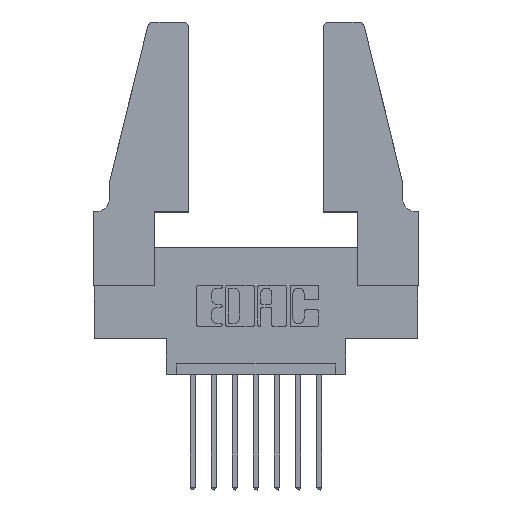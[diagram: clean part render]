
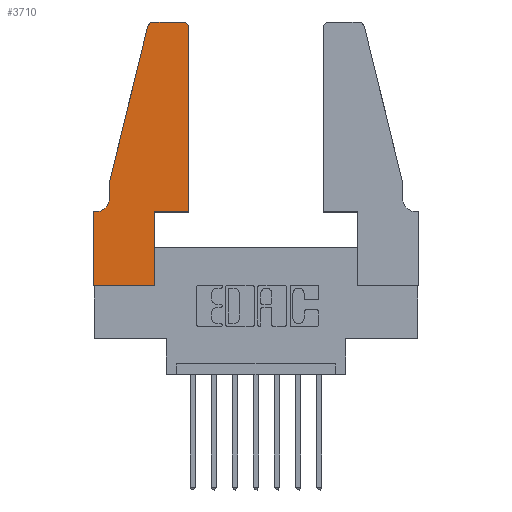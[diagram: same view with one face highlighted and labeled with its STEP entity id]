
A CAD part, top view. The second image highlights one B-rep face of the part: STEP entity #3710.
In plain terms, the highlighted planar face has unit normal (0, 0, 1).
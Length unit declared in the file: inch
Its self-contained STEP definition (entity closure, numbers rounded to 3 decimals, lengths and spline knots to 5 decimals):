
#387 = CARTESIAN_POINT ( 'NONE',  ( 0.2605, 1.25, 0.37 ) ) ;
#394 = DIRECTION ( 'NONE',  ( 1., 0., 0. ) ) ;
#398 = DIRECTION ( 'NONE',  ( -1., 0., 0. ) ) ;
#434 = ORIENTED_EDGE ( 'NONE', *, *, #7941, .T. ) ;
#473 = DIRECTION ( 'NONE',  ( -1., 0., 0. ) ) ;
#725 = ORIENTED_EDGE ( 'NONE', *, *, #10678, .T. ) ;
#937 = LINE ( 'NONE', #3140, #10698 ) ;
#984 = CARTESIAN_POINT ( 'NONE',  ( 0.0055, 0.35, 0.37 ) ) ;
#1072 = ORIENTED_EDGE ( 'NONE', *, *, #9021, .T. ) ;
#1118 = CARTESIAN_POINT ( 'NONE',  ( 0.4505, 0.35, 0.37 ) ) ;
#1166 = EDGE_CURVE ( 'NONE', #5108, #5320, #11151, .T. ) ;
#1177 = DIRECTION ( 'NONE',  ( 1., 0., 0. ) ) ;
#1738 = VERTEX_POINT ( 'NONE', #3221 ) ;
#1789 = LINE ( 'NONE', #6639, #7860 ) ;
#2050 = AXIS2_PLACEMENT_3D ( 'NONE', #4840, #11587, #1177 ) ;
#2088 = CARTESIAN_POINT ( 'NONE',  ( 0.0755, 0.5, 0.37 ) ) ;
#2323 = LINE ( 'NONE', #3815, #8827 ) ;
#2470 = ORIENTED_EDGE ( 'NONE', *, *, #11714, .T. ) ;
#2660 = CARTESIAN_POINT ( 'NONE',  ( 0.0055, 0.42, 0.37 ) ) ;
#2828 = EDGE_CURVE ( 'NONE', #4192, #9817, #10665, .T. ) ;
#2891 = VECTOR ( 'NONE', #8837, 39.37008 ) ;
#2918 = PLANE ( 'NONE',  #8118 ) ;
#3140 = CARTESIAN_POINT ( 'NONE',  ( 0.2865, 0.35, 0.37 ) ) ;
#3221 = CARTESIAN_POINT ( 'NONE',  ( 0.4505, 0.35, 0.37 ) ) ;
#3258 = CARTESIAN_POINT ( 'NONE',  ( 0.0755, 0.35, 0.37 ) ) ;
#3305 = CARTESIAN_POINT ( 'NONE',  ( 0.4205, 1.22, 0.37 ) ) ;
#3390 = ORIENTED_EDGE ( 'NONE', *, *, #5699, .T. ) ;
#3616 = DIRECTION ( 'NONE',  ( 0., 0., -1. ) ) ;
#3710 = ADVANCED_FACE ( 'NONE', ( #12267 ), #2918, .T. ) ;
#3715 = DIRECTION ( 'NONE',  ( 0., 0., 1. ) ) ;
#3815 = CARTESIAN_POINT ( 'NONE',  ( 0.4505, 0.35, 0.37 ) ) ;
#3877 = DIRECTION ( 'NONE',  ( 0., -1., 0. ) ) ;
#3938 = VECTOR ( 'NONE', #5956, 39.37008 ) ;
#4047 = LINE ( 'NONE', #3258, #8032 ) ;
#4055 = VECTOR ( 'NONE', #3877, 39.37008 ) ;
#4192 = VERTEX_POINT ( 'NONE', #7525 ) ;
#4229 = DIRECTION ( 'NONE',  ( 0., 0., 1. ) ) ;
#4243 = CARTESIAN_POINT ( 'NONE',  ( 0.2865, 0.35, 0.37 ) ) ;
#4402 = DIRECTION ( 'NONE',  ( 1., 0., 0. ) ) ;
#4688 = CARTESIAN_POINT ( 'NONE',  ( 0., 0.35, 0.37 ) ) ;
#4779 = LINE ( 'NONE', #1118, #11904 ) ;
#4840 = CARTESIAN_POINT ( 'NONE',  ( 0.284, 1.22, 0.37 ) ) ;
#4851 = DIRECTION ( 'NONE',  ( 1., 0., 0. ) ) ;
#5108 = VERTEX_POINT ( 'NONE', #7011 ) ;
#5204 = ORIENTED_EDGE ( 'NONE', *, *, #6131, .T. ) ;
#5320 = VERTEX_POINT ( 'NONE', #11475 ) ;
#5574 = CARTESIAN_POINT ( 'NONE',  ( 0.284, 1.25, 0.37 ) ) ;
#5699 = EDGE_CURVE ( 'NONE', #10253, #11839, #9743, .T. ) ;
#5833 = EDGE_CURVE ( 'NONE', #7370, #1738, #2323, .T. ) ;
#5854 = LINE ( 'NONE', #387, #10015 ) ;
#5956 = DIRECTION ( 'NONE',  ( 0., -1., 0. ) ) ;
#6131 = EDGE_CURVE ( 'NONE', #8356, #9611, #7935, .T. ) ;
#6154 = CARTESIAN_POINT ( 'NONE',  ( 0.0755, 0.5, 0.37 ) ) ;
#6639 = CARTESIAN_POINT ( 'NONE',  ( 0., 0., 0.37 ) ) ;
#7011 = CARTESIAN_POINT ( 'NONE',  ( 0.4505, 1.22, 0.37 ) ) ;
#7370 = VERTEX_POINT ( 'NONE', #4243 ) ;
#7496 = EDGE_LOOP ( 'NONE', ( #725, #1072, #3390, #10555, #10781, #434, #5204, #10088, #10394, #9271, #2470, #8524 ) ) ;
#7525 = CARTESIAN_POINT ( 'NONE',  ( 0.0755, 0.42, 0.37 ) ) ;
#7595 = LINE ( 'NONE', #8597, #4055 ) ;
#7598 = CARTESIAN_POINT ( 'NONE',  ( 0., 0.35, 0.37 ) ) ;
#7719 = DIRECTION ( 'NONE',  ( 0., 1., 0. ) ) ;
#7860 = VECTOR ( 'NONE', #4851, 39.37008 ) ;
#7924 = EDGE_CURVE ( 'NONE', #8750, #7370, #937, .T. ) ;
#7935 = LINE ( 'NONE', #10672, #3938 ) ;
#7941 = EDGE_CURVE ( 'NONE', #9817, #8356, #4047, .T. ) ;
#8032 = VECTOR ( 'NONE', #398, 39.37008 ) ;
#8035 = DIRECTION ( 'NONE',  ( 1., 0., 0. ) ) ;
#8118 = AXIS2_PLACEMENT_3D ( 'NONE', #7598, #3715, #394 ) ;
#8335 = VERTEX_POINT ( 'NONE', #5574 ) ;
#8356 = VERTEX_POINT ( 'NONE', #4688 ) ;
#8463 = EDGE_CURVE ( 'NONE', #9611, #8750, #1789, .T. ) ;
#8524 = ORIENTED_EDGE ( 'NONE', *, *, #1166, .T. ) ;
#8597 = CARTESIAN_POINT ( 'NONE',  ( 0.0755, 0.5, 0.37 ) ) ;
#8684 = DIRECTION ( 'NONE',  ( -1., 0., 0. ) ) ;
#8750 = VERTEX_POINT ( 'NONE', #11808 ) ;
#8818 = AXIS2_PLACEMENT_3D ( 'NONE', #2660, #3616, #8684 ) ;
#8827 = VECTOR ( 'NONE', #8035, 39.37008 ) ;
#8837 = DIRECTION ( 'NONE',  ( -0.239, -0.971, 0. ) ) ;
#8845 = DIRECTION ( 'NONE',  ( 0., 1., 0. ) ) ;
#9021 = EDGE_CURVE ( 'NONE', #8335, #10253, #10666, .T. ) ;
#9271 = ORIENTED_EDGE ( 'NONE', *, *, #5833, .T. ) ;
#9611 = VERTEX_POINT ( 'NONE', #10576 ) ;
#9743 = LINE ( 'NONE', #6154, #2891 ) ;
#9817 = VERTEX_POINT ( 'NONE', #984 ) ;
#10015 = VECTOR ( 'NONE', #473, 39.37008 ) ;
#10088 = ORIENTED_EDGE ( 'NONE', *, *, #8463, .T. ) ;
#10253 = VERTEX_POINT ( 'NONE', #12115 ) ;
#10394 = ORIENTED_EDGE ( 'NONE', *, *, #7924, .T. ) ;
#10555 = ORIENTED_EDGE ( 'NONE', *, *, #11786, .T. ) ;
#10576 = CARTESIAN_POINT ( 'NONE',  ( 0., 0., 0.37 ) ) ;
#10665 = CIRCLE ( 'NONE', #8818, 0.07 ) ;
#10666 = CIRCLE ( 'NONE', #2050, 0.03 ) ;
#10672 = CARTESIAN_POINT ( 'NONE',  ( 0., 0., 0.37 ) ) ;
#10678 = EDGE_CURVE ( 'NONE', #5320, #8335, #5854, .T. ) ;
#10698 = VECTOR ( 'NONE', #8845, 39.37008 ) ;
#10781 = ORIENTED_EDGE ( 'NONE', *, *, #2828, .T. ) ;
#11151 = CIRCLE ( 'NONE', #11731, 0.03 ) ;
#11475 = CARTESIAN_POINT ( 'NONE',  ( 0.4205, 1.25, 0.37 ) ) ;
#11587 = DIRECTION ( 'NONE',  ( 0., 0., 1. ) ) ;
#11714 = EDGE_CURVE ( 'NONE', #1738, #5108, #4779, .T. ) ;
#11731 = AXIS2_PLACEMENT_3D ( 'NONE', #3305, #4229, #4402 ) ;
#11786 = EDGE_CURVE ( 'NONE', #11839, #4192, #7595, .T. ) ;
#11808 = CARTESIAN_POINT ( 'NONE',  ( 0.2865, 0., 0.37 ) ) ;
#11839 = VERTEX_POINT ( 'NONE', #2088 ) ;
#11904 = VECTOR ( 'NONE', #7719, 39.37008 ) ;
#12115 = CARTESIAN_POINT ( 'NONE',  ( 0.25487, 1.22718, 0.37 ) ) ;
#12267 = FACE_OUTER_BOUND ( 'NONE', #7496, .T. ) ;
